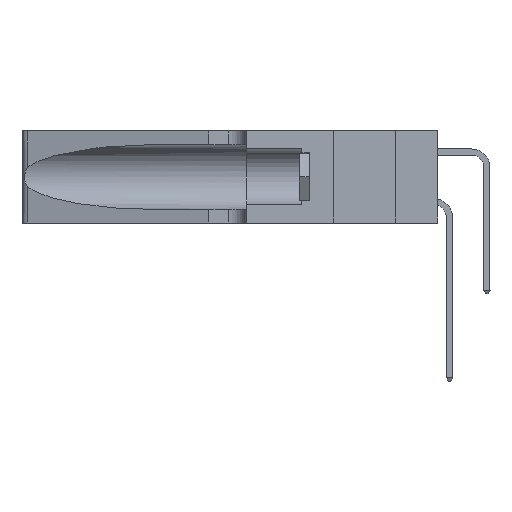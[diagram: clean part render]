
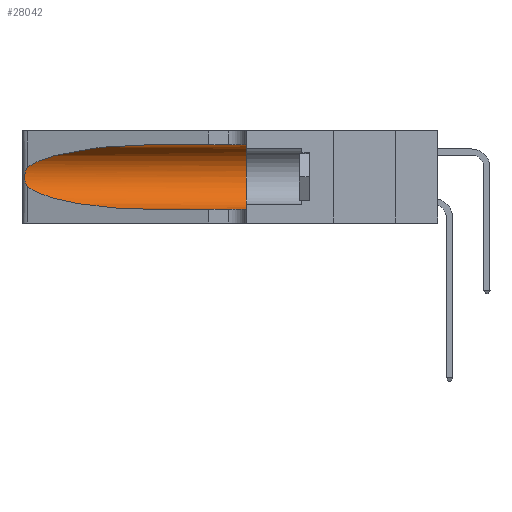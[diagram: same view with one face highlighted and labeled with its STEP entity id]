
A CAD part, left-side view. The second image highlights one B-rep face of the part: STEP entity #28042.
In plain terms, the highlighted cylindrical face has radius 3.308 mm (diameter 6.617 mm), a partial arc.
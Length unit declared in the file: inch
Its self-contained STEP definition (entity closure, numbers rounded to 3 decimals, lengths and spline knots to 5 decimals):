
#195 = CARTESIAN_POINT ( 'NONE',  ( 0.1305, 0.72297, 0.05475 ) ) ;
#659 = CARTESIAN_POINT ( 'NONE',  ( 0.25555, 1.22994, 0.2215 ) ) ;
#806 = CARTESIAN_POINT ( 'NONE',  ( 0.25789, 1.23486, 0.15765 ) ) ;
#838 = EDGE_CURVE ( 'NONE', #5033, #30664, #17108, .T. ) ;
#1520 = CARTESIAN_POINT ( 'NONE',  ( 0.1305, 0.35, 0.31525 ) ) ;
#1864 = VERTEX_POINT ( 'NONE', #3801 ) ;
#2158 = CARTESIAN_POINT ( 'NONE',  ( 0.18966, 0.96281, 0.31525 ) ) ;
#2343 = ORIENTED_EDGE ( 'NONE', *, *, #21636, .F. ) ;
#3801 = CARTESIAN_POINT ( 'NONE',  ( 0.25487, 1.22718, 0.22369 ) ) ;
#4103 = CARTESIAN_POINT ( 'NONE',  ( 0.25555, 1.22993, 0.14849 ) ) ;
#4684 = DIRECTION ( 'NONE',  ( 0., 1., 0. ) ) ;
#5033 = VERTEX_POINT ( 'NONE', #17722 ) ;
#5395 = CARTESIAN_POINT ( 'NONE',  ( 0.2373, 1.15595, 0.28018 ) ) ;
#7543 = VECTOR ( 'NONE', #26116, 39.37008 ) ;
#8875 = FACE_OUTER_BOUND ( 'NONE', #37715, .T. ) ;
#9103 = CARTESIAN_POINT ( 'NONE',  ( 0.1305, 0.35, 0.05475 ) ) ;
#9570 = LINE ( 'NONE', #18735, #17140 ) ;
#9653 = EDGE_CURVE ( 'NONE', #28254, #32821, #30951, .T. ) ;
#10229 = CARTESIAN_POINT ( 'NONE',  ( 0.25487, 1.22718, 0.22369 ) ) ;
#10370 = CARTESIAN_POINT ( 'NONE',  ( 0.25787, 1.23484, 0.2124 ) ) ;
#10863 = CARTESIAN_POINT ( 'NONE',  ( 0.1305, 1.61858, 0.185 ) ) ;
#13600 = CARTESIAN_POINT ( 'NONE',  ( 0.26018, 1.23835, 0.19895 ) ) ;
#13953 = EDGE_CURVE ( 'NONE', #32821, #39295, #9570, .T. ) ;
#14094 = DIRECTION ( 'NONE',  ( 0., 0., -1. ) ) ;
#14417 = CARTESIAN_POINT ( 'NONE',  ( 0.25487, 1.22718, 0.14631 ) ) ;
#14418 = ORIENTED_EDGE ( 'NONE', *, *, #838, .F. ) ;
#14875 = EDGE_CURVE ( 'NONE', #1864, #28254, #27918, .T. ) ;
#14940 = CARTESIAN_POINT ( 'NONE',  ( 0.25487, 1.22718, 0.14631 ) ) ;
#16850 = CARTESIAN_POINT ( 'NONE',  ( 0.26075, 1.23896, 0.178 ) ) ;
#17108 = LINE ( 'NONE', #28977, #7543 ) ;
#17140 = VECTOR ( 'NONE', #37881, 39.37008 ) ;
#17635 = EDGE_CURVE ( 'NONE', #5033, #1864, #20506, .T. ) ;
#17722 = CARTESIAN_POINT ( 'NONE',  ( 0.1305, 0.72297, 0.31525 ) ) ;
#18735 = CARTESIAN_POINT ( 'NONE',  ( 0.1305, 1.61858, 0.05475 ) ) ;
#20105 = CARTESIAN_POINT ( 'NONE',  ( 0.25856, 1.23593, 0.16098 ) ) ;
#20506 =( BOUNDED_CURVE ( )  B_SPLINE_CURVE ( 3, ( #21421, #2158, #5395, #27837 ),
 .UNSPECIFIED., .F., .F. ) 
 B_SPLINE_CURVE_WITH_KNOTS ( ( 4, 4 ),
 ( 1.5708, 2.84003 ),
 .UNSPECIFIED. ) 
 CURVE ( )  GEOMETRIC_REPRESENTATION_ITEM ( )  RATIONAL_B_SPLINE_CURVE ( ( 1., 0.87, 0.87, 1. ) ) 
 REPRESENTATION_ITEM ( '' )  );
#21421 = CARTESIAN_POINT ( 'NONE',  ( 0.1305, 0.72297, 0.31525 ) ) ;
#21636 = EDGE_CURVE ( 'NONE', #30664, #39295, #40642, .T. ) ;
#22562 = ORIENTED_EDGE ( 'NONE', *, *, #9653, .T. ) ;
#23305 = CARTESIAN_POINT ( 'NONE',  ( 0.25639, 1.23186, 0.15144 ) ) ;
#23909 = CARTESIAN_POINT ( 'NONE',  ( 0.1305, 0.35, 0.185 ) ) ;
#23946 = CYLINDRICAL_SURFACE ( 'NONE', #30510, 0.13025 ) ;
#24104 = ORIENTED_EDGE ( 'NONE', *, *, #14875, .T. ) ;
#26116 = DIRECTION ( 'NONE',  ( 0., -1., 0. ) ) ;
#26518 = CARTESIAN_POINT ( 'NONE',  ( 0.25487, 1.22718, 0.14631 ) ) ;
#27132 = DIRECTION ( 'NONE',  ( 0., 0., 1. ) ) ;
#27183 = AXIS2_PLACEMENT_3D ( 'NONE', #23909, #4684, #27132 ) ;
#27837 = CARTESIAN_POINT ( 'NONE',  ( 0.25487, 1.22718, 0.22369 ) ) ;
#27918 = B_SPLINE_CURVE_WITH_KNOTS ( 'NONE', 3,
 ( #10229, #659, #29563, #10370, #32764, #13600, #35967, #16850, #39208, #20105, #806, #23305, #4103, #26518 ),
 .UNSPECIFIED., .F., .F.,
 ( 4, 2, 2, 2, 2, 2, 4 ),
 ( 0., 0.00027, 0.00053, 0.00107, 0.0016, 0.00187, 0.00214 ),
 .UNSPECIFIED. ) ;
#28042 = ADVANCED_FACE ( 'NONE', ( #8875 ), #23946, .F. ) ;
#28254 = VERTEX_POINT ( 'NONE', #14940 ) ;
#28977 = CARTESIAN_POINT ( 'NONE',  ( 0.1305, 1.61858, 0.31525 ) ) ;
#29563 = CARTESIAN_POINT ( 'NONE',  ( 0.25639, 1.23184, 0.21858 ) ) ;
#30362 = CARTESIAN_POINT ( 'NONE',  ( 0.2373, 1.15595, 0.08982 ) ) ;
#30510 = AXIS2_PLACEMENT_3D ( 'NONE', #10863, #33229, #14094 ) ;
#30664 = VERTEX_POINT ( 'NONE', #1520 ) ;
#30951 =( BOUNDED_CURVE ( )  B_SPLINE_CURVE ( 3, ( #14417, #30362, #33549, #36774 ),
 .UNSPECIFIED., .F., .F. ) 
 B_SPLINE_CURVE_WITH_KNOTS ( ( 4, 4 ),
 ( 3.44316, 4.71239 ),
 .UNSPECIFIED. ) 
 CURVE ( )  GEOMETRIC_REPRESENTATION_ITEM ( )  RATIONAL_B_SPLINE_CURVE ( ( 1., 0.87, 0.87, 1. ) ) 
 REPRESENTATION_ITEM ( '' )  );
#32231 = ORIENTED_EDGE ( 'NONE', *, *, #13953, .T. ) ;
#32764 = CARTESIAN_POINT ( 'NONE',  ( 0.25854, 1.2359, 0.20912 ) ) ;
#32821 = VERTEX_POINT ( 'NONE', #195 ) ;
#33229 = DIRECTION ( 'NONE',  ( 0., -1., 0. ) ) ;
#33549 = CARTESIAN_POINT ( 'NONE',  ( 0.18966, 0.96281, 0.05475 ) ) ;
#35967 = CARTESIAN_POINT ( 'NONE',  ( 0.26075, 1.23896, 0.19203 ) ) ;
#36774 = CARTESIAN_POINT ( 'NONE',  ( 0.1305, 0.72297, 0.05475 ) ) ;
#37186 = ORIENTED_EDGE ( 'NONE', *, *, #17635, .T. ) ;
#37715 = EDGE_LOOP ( 'NONE', ( #37186, #24104, #22562, #32231, #2343, #14418 ) ) ;
#37881 = DIRECTION ( 'NONE',  ( 0., -1., 0. ) ) ;
#39208 = CARTESIAN_POINT ( 'NONE',  ( 0.26017, 1.23833, 0.17102 ) ) ;
#39295 = VERTEX_POINT ( 'NONE', #9103 ) ;
#40642 = CIRCLE ( 'NONE', #27183, 0.13025 ) ;
